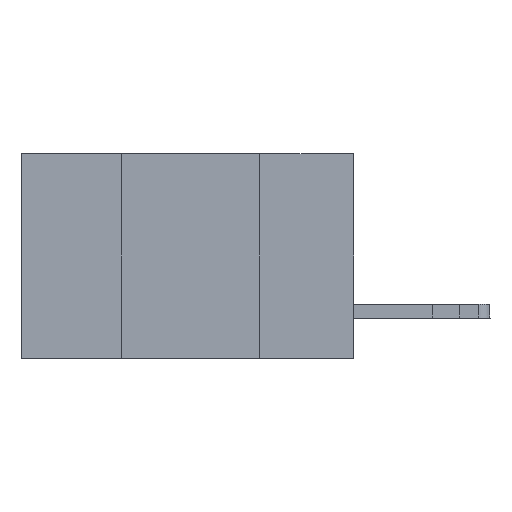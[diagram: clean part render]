
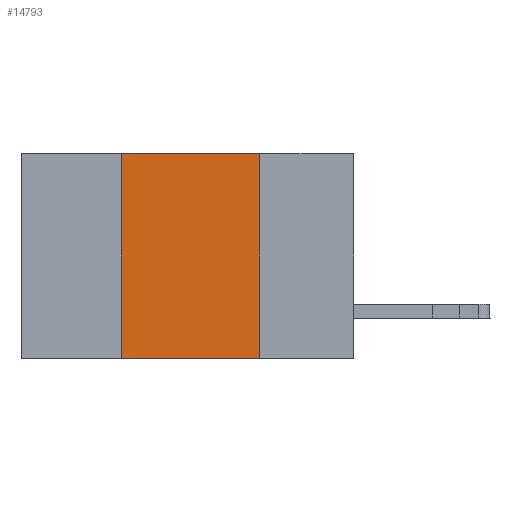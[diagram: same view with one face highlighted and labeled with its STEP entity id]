
A CAD part, left-side view. The second image highlights one B-rep face of the part: STEP entity #14793.
In plain terms, the highlighted planar face has unit normal (-1, 0, 0).
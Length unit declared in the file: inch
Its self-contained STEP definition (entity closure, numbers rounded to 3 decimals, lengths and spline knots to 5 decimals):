
#487 = VECTOR ( 'NONE', #23222, 39.37008 ) ;
#1268 = PLANE ( 'NONE',  #15458 ) ;
#1300 = DIRECTION ( 'NONE',  ( 0., 0., 1. ) ) ;
#1357 = DIRECTION ( 'NONE',  ( 1., 0., 0. ) ) ;
#1554 = LINE ( 'NONE', #20472, #8472 ) ;
#2739 = CARTESIAN_POINT ( 'NONE',  ( 0., 0.42, 0. ) ) ;
#2975 = VERTEX_POINT ( 'NONE', #10976 ) ;
#4278 = FACE_OUTER_BOUND ( 'NONE', #25409, .T. ) ;
#4542 = VERTEX_POINT ( 'NONE', #2739 ) ;
#5683 = VECTOR ( 'NONE', #10282, 39.37008 ) ;
#7468 = CARTESIAN_POINT ( 'NONE',  ( 0., 0.6, -0.37 ) ) ;
#7622 = ORIENTED_EDGE ( 'NONE', *, *, #9014, .T. ) ;
#7665 = VECTOR ( 'NONE', #1300, 39.37008 ) ;
#8137 = ORIENTED_EDGE ( 'NONE', *, *, #24000, .F. ) ;
#8472 = VECTOR ( 'NONE', #25042, 39.37008 ) ;
#8957 = VERTEX_POINT ( 'NONE', #24799 ) ;
#9014 = EDGE_CURVE ( 'NONE', #2975, #8957, #15640, .T. ) ;
#10282 = DIRECTION ( 'NONE',  ( 0., -1., 0. ) ) ;
#10434 = CARTESIAN_POINT ( 'NONE',  ( 0., 0.17, 0. ) ) ;
#10976 = CARTESIAN_POINT ( 'NONE',  ( 0., 0.42, -0.37 ) ) ;
#12643 = EDGE_CURVE ( 'NONE', #4542, #14029, #21741, .T. ) ;
#13418 = CARTESIAN_POINT ( 'NONE',  ( 0., 0.6, 0. ) ) ;
#14029 = VERTEX_POINT ( 'NONE', #10434 ) ;
#14793 = ADVANCED_FACE ( 'NONE', ( #4278 ), #1268, .F. ) ;
#15458 = AXIS2_PLACEMENT_3D ( 'NONE', #13418, #1357, #15527 ) ;
#15527 = DIRECTION ( 'NONE',  ( 0., 0., -1. ) ) ;
#15640 = LINE ( 'NONE', #7468, #487 ) ;
#17603 = CARTESIAN_POINT ( 'NONE',  ( 0., 0.42, 0. ) ) ;
#18407 = CARTESIAN_POINT ( 'NONE',  ( 0., 0.6, 0. ) ) ;
#20472 = CARTESIAN_POINT ( 'NONE',  ( 0., 0.17, 0. ) ) ;
#21741 = LINE ( 'NONE', #18407, #5683 ) ;
#22099 = ORIENTED_EDGE ( 'NONE', *, *, #12643, .F. ) ;
#23222 = DIRECTION ( 'NONE',  ( 0., -1., 0. ) ) ;
#24000 = EDGE_CURVE ( 'NONE', #14029, #8957, #1554, .T. ) ;
#24375 = LINE ( 'NONE', #17603, #7665 ) ;
#24799 = CARTESIAN_POINT ( 'NONE',  ( 0., 0.17, -0.37 ) ) ;
#25042 = DIRECTION ( 'NONE',  ( 0., 0., -1. ) ) ;
#25409 = EDGE_LOOP ( 'NONE', ( #8137, #22099, #25602, #7622 ) ) ;
#25568 = EDGE_CURVE ( 'NONE', #2975, #4542, #24375, .T. ) ;
#25602 = ORIENTED_EDGE ( 'NONE', *, *, #25568, .F. ) ;
